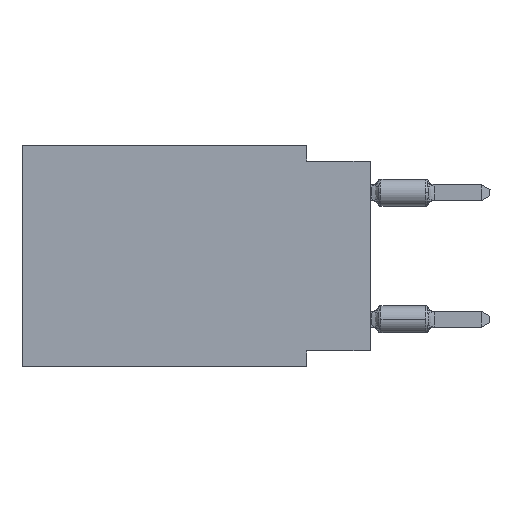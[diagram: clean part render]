
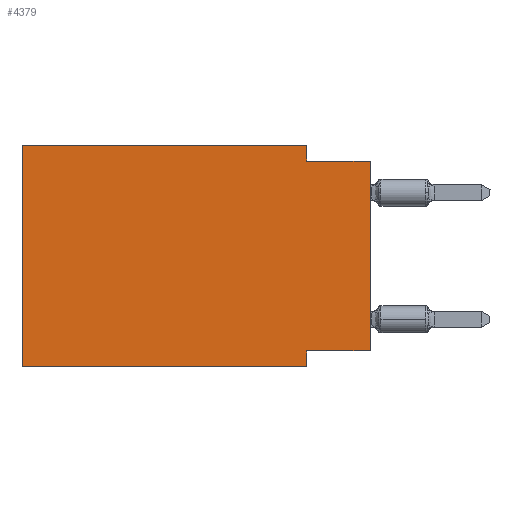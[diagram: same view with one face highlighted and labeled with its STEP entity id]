
A CAD part, left-side view. The second image highlights one B-rep face of the part: STEP entity #4379.
In plain terms, the highlighted planar face has unit normal (-1, 0, 0).
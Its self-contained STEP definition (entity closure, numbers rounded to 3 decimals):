
#1163 = VERTEX_POINT ( 'NONE', #61517 ) ;
#1353 = CARTESIAN_POINT ( 'NONE',  ( 0., 13.97, -8.89 ) ) ;
#1843 = ORIENTED_EDGE ( 'NONE', *, *, #33767, .T. ) ;
#2691 = DIRECTION ( 'NONE',  ( 0., 0., 1. ) ) ;
#4346 = VERTEX_POINT ( 'NONE', #61443 ) ;
#4379 = ADVANCED_FACE ( 'NONE', ( #50105 ), #6219, .F. ) ;
#6219 = PLANE ( 'NONE',  #48844 ) ;
#6417 = DIRECTION ( 'NONE',  ( 0., -1., 0. ) ) ;
#6792 = CARTESIAN_POINT ( 'NONE',  ( 0., 13.97, -8.89 ) ) ;
#10697 = CARTESIAN_POINT ( 'NONE',  ( 0., 2.54, -8.89 ) ) ;
#11407 = VERTEX_POINT ( 'NONE', #43972 ) ;
#12236 = LINE ( 'NONE', #21126, #39980 ) ;
#12770 = DIRECTION ( 'NONE',  ( 0., 0., -1. ) ) ;
#13761 = LINE ( 'NONE', #38251, #44750 ) ;
#15939 = LINE ( 'NONE', #1353, #45494 ) ;
#16407 = CARTESIAN_POINT ( 'NONE',  ( 0., 2.54, -8.255 ) ) ;
#20383 = EDGE_LOOP ( 'NONE', ( #1843, #31251, #22080, #56060, #58172, #61088, #61622, #51280 ) ) ;
#20386 = EDGE_CURVE ( 'NONE', #59450, #11407, #31368, .T. ) ;
#20556 = CARTESIAN_POINT ( 'NONE',  ( 0., 13.97, 0. ) ) ;
#21126 = CARTESIAN_POINT ( 'NONE',  ( 0., 0., 0. ) ) ;
#22080 = ORIENTED_EDGE ( 'NONE', *, *, #55620, .F. ) ;
#22325 = LINE ( 'NONE', #45556, #24742 ) ;
#22649 = VERTEX_POINT ( 'NONE', #16407 ) ;
#23749 = LINE ( 'NONE', #32994, #48784 ) ;
#23998 = CARTESIAN_POINT ( 'NONE',  ( 0., 2.54, 0. ) ) ;
#24742 = VECTOR ( 'NONE', #12770, 1000. ) ;
#25918 = DIRECTION ( 'NONE',  ( 0., 0., -1. ) ) ;
#25953 = EDGE_CURVE ( 'NONE', #22649, #40026, #38878, .T. ) ;
#28719 = DIRECTION ( 'NONE',  ( 0., 1., 0. ) ) ;
#29961 = DIRECTION ( 'NONE',  ( 0., 0., -1. ) ) ;
#30390 = LINE ( 'NONE', #31646, #60266 ) ;
#30709 = DIRECTION ( 'NONE',  ( 0., -1., 0. ) ) ;
#30794 = VERTEX_POINT ( 'NONE', #61161 ) ;
#31251 = ORIENTED_EDGE ( 'NONE', *, *, #33729, .F. ) ;
#31368 = LINE ( 'NONE', #20556, #32462 ) ;
#31646 = CARTESIAN_POINT ( 'NONE',  ( 0., 0., -0.635 ) ) ;
#32462 = VECTOR ( 'NONE', #55548, 1000. ) ;
#32994 = CARTESIAN_POINT ( 'NONE',  ( 0., 13.97, 0. ) ) ;
#33729 = EDGE_CURVE ( 'NONE', #1163, #30794, #30390, .T. ) ;
#33767 = EDGE_CURVE ( 'NONE', #4346, #30794, #12236, .T. ) ;
#35264 = EDGE_CURVE ( 'NONE', #4346, #22649, #13761, .T. ) ;
#38251 = CARTESIAN_POINT ( 'NONE',  ( 0., 0., -8.255 ) ) ;
#38878 = LINE ( 'NONE', #43330, #56797 ) ;
#39980 = VECTOR ( 'NONE', #2691, 1000. ) ;
#40026 = VERTEX_POINT ( 'NONE', #10697 ) ;
#43330 = CARTESIAN_POINT ( 'NONE',  ( 0., 2.54, -8.89 ) ) ;
#43972 = CARTESIAN_POINT ( 'NONE',  ( 0., 13.97, 0. ) ) ;
#44704 = CARTESIAN_POINT ( 'NONE',  ( 0., 13.97, 0. ) ) ;
#44750 = VECTOR ( 'NONE', #28719, 1000. ) ;
#45494 = VECTOR ( 'NONE', #6417, 1000. ) ;
#45556 = CARTESIAN_POINT ( 'NONE',  ( 0., 2.54, 0. ) ) ;
#48784 = VECTOR ( 'NONE', #52398, 1000. ) ;
#48844 = AXIS2_PLACEMENT_3D ( 'NONE', #44704, #49797, #25918 ) ;
#49797 = DIRECTION ( 'NONE',  ( 1., 0., 0. ) ) ;
#50105 = FACE_OUTER_BOUND ( 'NONE', #20383, .T. ) ;
#50247 = VERTEX_POINT ( 'NONE', #23998 ) ;
#51280 = ORIENTED_EDGE ( 'NONE', *, *, #35264, .F. ) ;
#52398 = DIRECTION ( 'NONE',  ( 0., -1., 0. ) ) ;
#55548 = DIRECTION ( 'NONE',  ( 0., 0., 1. ) ) ;
#55620 = EDGE_CURVE ( 'NONE', #50247, #1163, #22325, .T. ) ;
#56060 = ORIENTED_EDGE ( 'NONE', *, *, #57663, .F. ) ;
#56797 = VECTOR ( 'NONE', #29961, 1000. ) ;
#57663 = EDGE_CURVE ( 'NONE', #11407, #50247, #23749, .T. ) ;
#58172 = ORIENTED_EDGE ( 'NONE', *, *, #20386, .F. ) ;
#59450 = VERTEX_POINT ( 'NONE', #6792 ) ;
#60266 = VECTOR ( 'NONE', #30709, 1000. ) ;
#61088 = ORIENTED_EDGE ( 'NONE', *, *, #61231, .T. ) ;
#61161 = CARTESIAN_POINT ( 'NONE',  ( 0., 0., -0.635 ) ) ;
#61231 = EDGE_CURVE ( 'NONE', #59450, #40026, #15939, .T. ) ;
#61443 = CARTESIAN_POINT ( 'NONE',  ( 0., 0., -8.255 ) ) ;
#61517 = CARTESIAN_POINT ( 'NONE',  ( 0., 2.54, -0.635 ) ) ;
#61622 = ORIENTED_EDGE ( 'NONE', *, *, #25953, .F. ) ;
